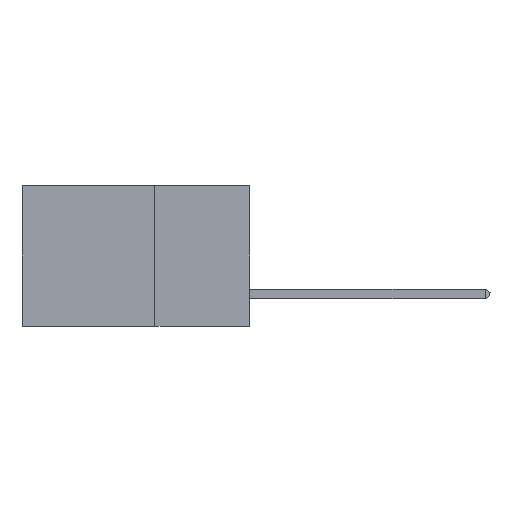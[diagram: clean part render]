
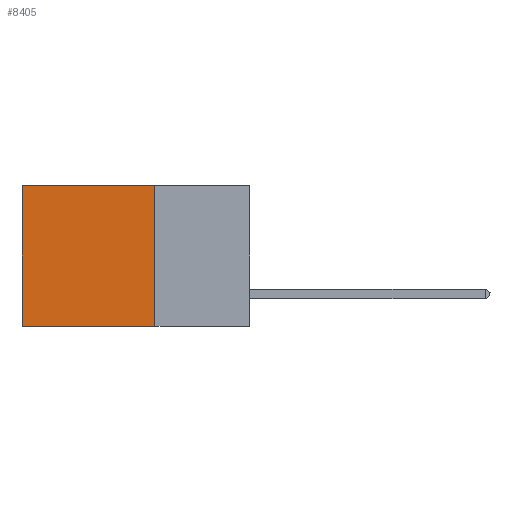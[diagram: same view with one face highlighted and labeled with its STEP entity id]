
A CAD part, left-side view. The second image highlights one B-rep face of the part: STEP entity #8405.
In plain terms, the highlighted planar face has unit normal (-1, 0, 0).
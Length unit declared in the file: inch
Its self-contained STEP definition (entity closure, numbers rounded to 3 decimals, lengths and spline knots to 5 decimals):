
#407 = VECTOR ( 'NONE', #4034, 39.37008 ) ;
#916 = CARTESIAN_POINT ( 'NONE',  ( 0.2875, 0.25, 0. ) ) ;
#1046 = LINE ( 'NONE', #9184, #6218 ) ;
#1341 = LINE ( 'NONE', #6107, #407 ) ;
#1847 = CARTESIAN_POINT ( 'NONE',  ( 0.2875, 0.25, 0. ) ) ;
#2829 = LINE ( 'NONE', #22109, #24685 ) ;
#3002 = CARTESIAN_POINT ( 'NONE',  ( 0.2875, 0.6, 0. ) ) ;
#3083 = PLANE ( 'NONE',  #12178 ) ;
#4034 = DIRECTION ( 'NONE',  ( 0., 1., 0. ) ) ;
#4421 = VERTEX_POINT ( 'NONE', #1847 ) ;
#4638 = CARTESIAN_POINT ( 'NONE',  ( 0.2875, 0.6, -0.37 ) ) ;
#5235 = DIRECTION ( 'NONE',  ( 0., 0., -1. ) ) ;
#6103 = ORIENTED_EDGE ( 'NONE', *, *, #19328, .T. ) ;
#6107 = CARTESIAN_POINT ( 'NONE',  ( 0.2875, 0.25, -0.37 ) ) ;
#6218 = VECTOR ( 'NONE', #9004, 39.37008 ) ;
#6472 = VERTEX_POINT ( 'NONE', #12632 ) ;
#6613 = VERTEX_POINT ( 'NONE', #4638 ) ;
#7130 = CARTESIAN_POINT ( 'NONE',  ( 0.2875, 0.25, 0. ) ) ;
#7220 = DIRECTION ( 'NONE',  ( 1., 0., 0. ) ) ;
#7904 = DIRECTION ( 'NONE',  ( 0., 0., -1. ) ) ;
#8405 = ADVANCED_FACE ( 'NONE', ( #15229 ), #3083, .F. ) ;
#9004 = DIRECTION ( 'NONE',  ( 0., 1., 0. ) ) ;
#9184 = CARTESIAN_POINT ( 'NONE',  ( 0.2875, 0.25, 0. ) ) ;
#10325 = VERTEX_POINT ( 'NONE', #3002 ) ;
#12178 = AXIS2_PLACEMENT_3D ( 'NONE', #7130, #7220, #23337 ) ;
#12632 = CARTESIAN_POINT ( 'NONE',  ( 0.2875, 0.25, -0.37 ) ) ;
#15229 = FACE_OUTER_BOUND ( 'NONE', #24455, .T. ) ;
#15455 = ORIENTED_EDGE ( 'NONE', *, *, #15704, .T. ) ;
#15704 = EDGE_CURVE ( 'NONE', #4421, #10325, #1046, .T. ) ;
#16518 = EDGE_CURVE ( 'NONE', #6472, #6613, #1341, .T. ) ;
#18226 = ORIENTED_EDGE ( 'NONE', *, *, #16518, .F. ) ;
#19328 = EDGE_CURVE ( 'NONE', #10325, #6613, #2829, .T. ) ;
#20103 = VECTOR ( 'NONE', #5235, 39.37008 ) ;
#20431 = EDGE_CURVE ( 'NONE', #4421, #6472, #25567, .T. ) ;
#22109 = CARTESIAN_POINT ( 'NONE',  ( 0.2875, 0.6, 0. ) ) ;
#23337 = DIRECTION ( 'NONE',  ( 0., 0., -1. ) ) ;
#24455 = EDGE_LOOP ( 'NONE', ( #6103, #18226, #25634, #15455 ) ) ;
#24685 = VECTOR ( 'NONE', #7904, 39.37008 ) ;
#25567 = LINE ( 'NONE', #916, #20103 ) ;
#25634 = ORIENTED_EDGE ( 'NONE', *, *, #20431, .F. ) ;
